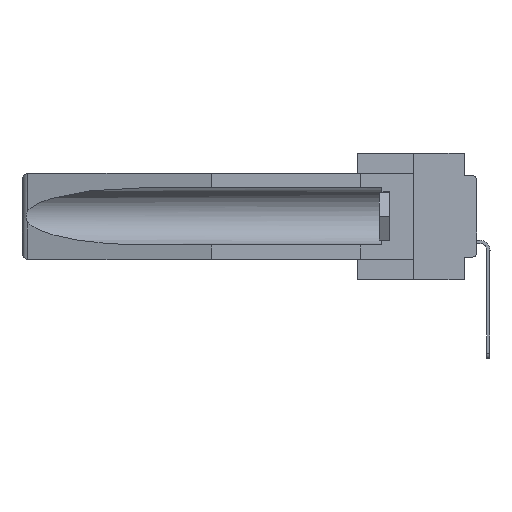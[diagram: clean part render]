
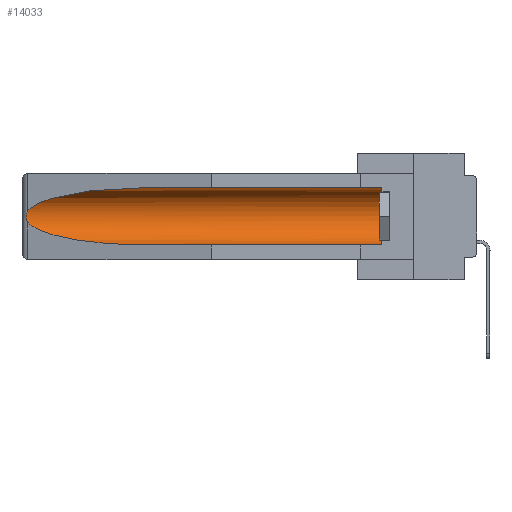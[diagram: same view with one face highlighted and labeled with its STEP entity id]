
A CAD part, left-side view. The second image highlights one B-rep face of the part: STEP entity #14033.
In plain terms, the highlighted cylindrical face has radius 2.857 mm (diameter 5.715 mm), a partial arc.
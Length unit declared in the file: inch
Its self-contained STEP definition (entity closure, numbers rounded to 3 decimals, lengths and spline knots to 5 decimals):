
#719 = CARTESIAN_POINT ( 'NONE',  ( 0.26537, 1.52718, -0.14972 ) ) ;
#838 = CARTESIAN_POINT ( 'NONE',  ( 0.155, 1.07973, -0.284 ) ) ;
#987 = CARTESIAN_POINT ( 'NONE',  ( 0.155, 0.126, -0.284 ) ) ;
#1076 = LINE ( 'NONE', #10110, #32793 ) ;
#1959 = VERTEX_POINT ( 'NONE', #34498 ) ;
#2335 = DIRECTION ( 'NONE',  ( 0., 0., 1. ) ) ;
#2343 = CARTESIAN_POINT ( 'NONE',  ( 0.2675, 1.53308, -0.17534 ) ) ;
#2483 = ORIENTED_EDGE ( 'NONE', *, *, #28254, .T. ) ;
#3119 = CARTESIAN_POINT ( 'NONE',  ( 0.155, 1.07973, -0.284 ) ) ;
#5215 = CARTESIAN_POINT ( 'NONE',  ( 0.26654, 1.53092, -0.15636 ) ) ;
#5404 = CARTESIAN_POINT ( 'NONE',  ( 0.155, 0.126, -0.1715 ) ) ;
#5411 = CARTESIAN_POINT ( 'NONE',  ( 0.26655, 1.53094, -0.18657 ) ) ;
#5514 = ORIENTED_EDGE ( 'NONE', *, *, #10374, .T. ) ;
#5837 = DIRECTION ( 'NONE',  ( 0., 0., 1. ) ) ;
#6152 = ORIENTED_EDGE ( 'NONE', *, *, #29626, .T. ) ;
#6975 = CIRCLE ( 'NONE', #17976, 0.1125 ) ;
#7293 = CARTESIAN_POINT ( 'NONE',  ( 0.25451, 1.48313, -0.09465 ) ) ;
#8295 = CARTESIAN_POINT ( 'NONE',  ( 0.26597, 1.52961, -0.15275 ) ) ;
#9845 = CARTESIAN_POINT ( 'NONE',  ( 0.21114, 1.30732, -0.284 ) ) ;
#10110 = CARTESIAN_POINT ( 'NONE',  ( 0.155, -0.30754, -0.059 ) ) ;
#10370 = CARTESIAN_POINT ( 'NONE',  ( 0.155, 1.07973, -0.059 ) ) ;
#10374 = EDGE_CURVE ( 'NONE', #1959, #15499, #31152, .T. ) ;
#10882 = CARTESIAN_POINT ( 'NONE',  ( 0.155, 0.126, -0.059 ) ) ;
#13858 = DIRECTION ( 'NONE',  ( 0., -1., 0. ) ) ;
#13866 = CARTESIAN_POINT ( 'NONE',  ( 0.26537, 1.52718, -0.14972 ) ) ;
#14033 = ADVANCED_FACE ( 'NONE', ( #31691 ), #22533, .F. ) ;
#14196 = CARTESIAN_POINT ( 'NONE',  ( 0.155, 1.07973, -0.059 ) ) ;
#15193 = CARTESIAN_POINT ( 'NONE',  ( 0.25451, 1.48313, -0.24835 ) ) ;
#15499 = VERTEX_POINT ( 'NONE', #838 ) ;
#16909 = CARTESIAN_POINT ( 'NONE',  ( 0.2673, 1.5327, -0.16383 ) ) ;
#17101 = CARTESIAN_POINT ( 'NONE',  ( 0.26597, 1.5296, -0.19026 ) ) ;
#17345 = CARTESIAN_POINT ( 'NONE',  ( 0.155, -0.30754, -0.1715 ) ) ;
#17976 = AXIS2_PLACEMENT_3D ( 'NONE', #5404, #13858, #2335 ) ;
#19171 = CARTESIAN_POINT ( 'NONE',  ( 0.26537, 1.52718, -0.14972 ) ) ;
#19337 = VECTOR ( 'NONE', #24583, 39.37008 ) ;
#19799 = EDGE_CURVE ( 'NONE', #20206, #15499, #21548, .T. ) ;
#19976 = CARTESIAN_POINT ( 'NONE',  ( 0.2673, 1.53269, -0.17917 ) ) ;
#20206 = VERTEX_POINT ( 'NONE', #987 ) ;
#21548 = LINE ( 'NONE', #33214, #19337 ) ;
#22044 = CARTESIAN_POINT ( 'NONE',  ( 0.21114, 1.30732, -0.059 ) ) ;
#22533 = CYLINDRICAL_SURFACE ( 'NONE', #34933, 0.1125 ) ;
#22663 = VERTEX_POINT ( 'NONE', #10882 ) ;
#23824 = VERTEX_POINT ( 'NONE', #719 ) ;
#24583 = DIRECTION ( 'NONE',  ( 0., 1., 0. ) ) ;
#25407 = EDGE_CURVE ( 'NONE', #30546, #23824, #32375, .T. ) ;
#26420 = EDGE_LOOP ( 'NONE', ( #32379, #6152, #5514, #26430, #2483, #27474 ) ) ;
#26430 = ORIENTED_EDGE ( 'NONE', *, *, #19799, .F. ) ;
#27474 = ORIENTED_EDGE ( 'NONE', *, *, #32285, .T. ) ;
#27489 = DIRECTION ( 'NONE',  ( 0., 1., 0. ) ) ;
#28254 = EDGE_CURVE ( 'NONE', #20206, #22663, #6975, .T. ) ;
#28571 = CARTESIAN_POINT ( 'NONE',  ( 0.2675, 1.53308, -0.16763 ) ) ;
#28754 = CARTESIAN_POINT ( 'NONE',  ( 0.26537, 1.52718, -0.19328 ) ) ;
#29626 = EDGE_CURVE ( 'NONE', #23824, #1959, #33975, .T. ) ;
#29921 = CARTESIAN_POINT ( 'NONE',  ( 0.26537, 1.52718, -0.19328 ) ) ;
#30546 = VERTEX_POINT ( 'NONE', #14196 ) ;
#31152 =( BOUNDED_CURVE ( )  B_SPLINE_CURVE ( 3, ( #29921, #15193, #9845, #3119 ),
 .UNSPECIFIED., .F., .F. ) 
 B_SPLINE_CURVE_WITH_KNOTS ( ( 4, 4 ),
 ( 0.1948, 1.5708 ),
 .UNSPECIFIED. ) 
 CURVE ( )  GEOMETRIC_REPRESENTATION_ITEM ( )  RATIONAL_B_SPLINE_CURVE ( ( 1., 0.848, 0.848, 1. ) ) 
 REPRESENTATION_ITEM ( '' )  );
#31691 = FACE_OUTER_BOUND ( 'NONE', #26420, .T. ) ;
#32285 = EDGE_CURVE ( 'NONE', #22663, #30546, #1076, .T. ) ;
#32375 =( BOUNDED_CURVE ( )  B_SPLINE_CURVE ( 3, ( #10370, #22044, #7293, #19171 ),
 .UNSPECIFIED., .F., .F. ) 
 B_SPLINE_CURVE_WITH_KNOTS ( ( 4, 4 ),
 ( 4.71239, 6.08839 ),
 .UNSPECIFIED. ) 
 CURVE ( )  GEOMETRIC_REPRESENTATION_ITEM ( )  RATIONAL_B_SPLINE_CURVE ( ( 1., 0.848, 0.848, 1. ) ) 
 REPRESENTATION_ITEM ( '' )  );
#32379 = ORIENTED_EDGE ( 'NONE', *, *, #25407, .T. ) ;
#32793 = VECTOR ( 'NONE', #27489, 39.37008 ) ;
#33214 = CARTESIAN_POINT ( 'NONE',  ( 0.155, -0.30754, -0.284 ) ) ;
#33975 = B_SPLINE_CURVE_WITH_KNOTS ( 'NONE', 3,
 ( #13866, #8295, #5215, #16909, #28571, #2343, #19976, #5411, #17101, #28754 ),
 .UNSPECIFIED., .F., .F.,
 ( 4, 2, 2, 2, 4 ),
 ( 0., 0.00029, 0.00058, 0.00087, 0.00117 ),
 .UNSPECIFIED. ) ;
#34498 = CARTESIAN_POINT ( 'NONE',  ( 0.26537, 1.52718, -0.19328 ) ) ;
#34564 = DIRECTION ( 'NONE',  ( 0., 1., 0. ) ) ;
#34933 = AXIS2_PLACEMENT_3D ( 'NONE', #17345, #34564, #5837 ) ;
